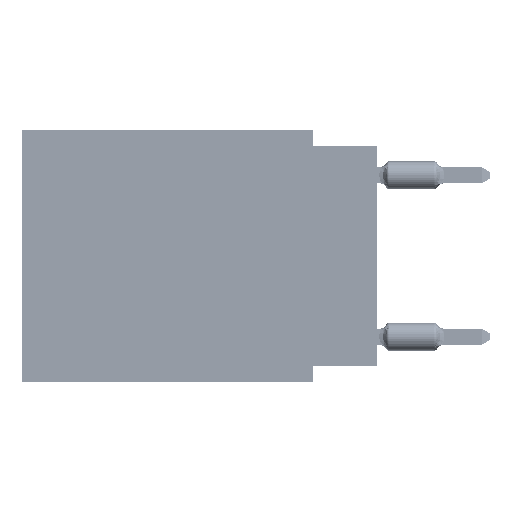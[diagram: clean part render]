
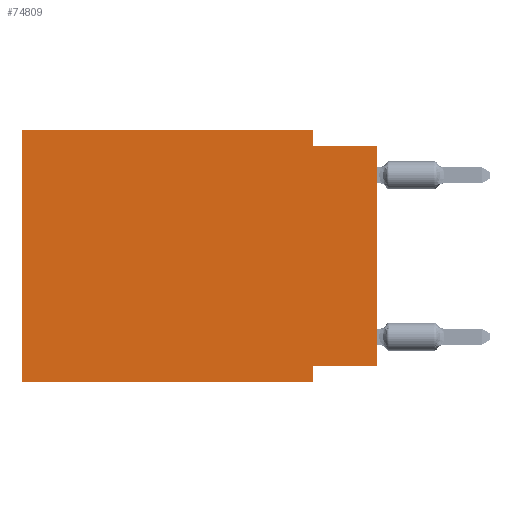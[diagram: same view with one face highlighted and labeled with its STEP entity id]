
A CAD part, left-side view. The second image highlights one B-rep face of the part: STEP entity #74809.
In plain terms, the highlighted planar face has unit normal (-1, 0, 0).
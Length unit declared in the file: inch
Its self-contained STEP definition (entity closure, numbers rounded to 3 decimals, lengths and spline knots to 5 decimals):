
#407 = CARTESIAN_POINT ( 'NONE',  ( 0., 0.1, -0.025 ) ) ;
#1064 = DIRECTION ( 'NONE',  ( 0., -1., 0. ) ) ;
#2382 = LINE ( 'NONE', #27603, #84519 ) ;
#2396 = FACE_OUTER_BOUND ( 'NONE', #12729, .T. ) ;
#2528 = CARTESIAN_POINT ( 'NONE',  ( 0., 0.1, -0.365 ) ) ;
#4672 = VECTOR ( 'NONE', #81144, 39.37008 ) ;
#7283 = CARTESIAN_POINT ( 'NONE',  ( 0., 0.55, -0.39 ) ) ;
#10676 = LINE ( 'NONE', #62419, #72088 ) ;
#12478 = DIRECTION ( 'NONE',  ( 0., -1., 0. ) ) ;
#12547 = VECTOR ( 'NONE', #30053, 39.37008 ) ;
#12703 = CARTESIAN_POINT ( 'NONE',  ( 0., 0.55, 0. ) ) ;
#12729 = EDGE_LOOP ( 'NONE', ( #14983, #24178, #57333, #37853, #65260, #55262, #60399, #20203 ) ) ;
#14983 = ORIENTED_EDGE ( 'NONE', *, *, #69082, .T. ) ;
#19561 = VERTEX_POINT ( 'NONE', #55172 ) ;
#20203 = ORIENTED_EDGE ( 'NONE', *, *, #21071, .F. ) ;
#20659 = PLANE ( 'NONE',  #43314 ) ;
#21071 = EDGE_CURVE ( 'NONE', #53853, #50099, #47751, .T. ) ;
#23182 = VERTEX_POINT ( 'NONE', #60669 ) ;
#24178 = ORIENTED_EDGE ( 'NONE', *, *, #59962, .F. ) ;
#25456 = VERTEX_POINT ( 'NONE', #407 ) ;
#27009 = CARTESIAN_POINT ( 'NONE',  ( 0., 0., -0.365 ) ) ;
#27603 = CARTESIAN_POINT ( 'NONE',  ( 0., 0., 0. ) ) ;
#28454 = EDGE_CURVE ( 'NONE', #53299, #55441, #10676, .T. ) ;
#28886 = DIRECTION ( 'NONE',  ( 1., 0., 0. ) ) ;
#29980 = EDGE_CURVE ( 'NONE', #55441, #23182, #59302, .T. ) ;
#30053 = DIRECTION ( 'NONE',  ( 0., 0., -1. ) ) ;
#30653 = VECTOR ( 'NONE', #1064, 39.37008 ) ;
#30919 = CARTESIAN_POINT ( 'NONE',  ( 0., 0.1, 0. ) ) ;
#37853 = ORIENTED_EDGE ( 'NONE', *, *, #29980, .F. ) ;
#38728 = LINE ( 'NONE', #85182, #50226 ) ;
#43126 = LINE ( 'NONE', #30919, #12547 ) ;
#43314 = AXIS2_PLACEMENT_3D ( 'NONE', #81021, #28886, #81879 ) ;
#43472 = VECTOR ( 'NONE', #12478, 39.37008 ) ;
#47751 = LINE ( 'NONE', #53809, #4672 ) ;
#50099 = VERTEX_POINT ( 'NONE', #2528 ) ;
#50226 = VECTOR ( 'NONE', #53479, 39.37008 ) ;
#53299 = VERTEX_POINT ( 'NONE', #69831 ) ;
#53479 = DIRECTION ( 'NONE',  ( 0., 0., -1. ) ) ;
#53782 = DIRECTION ( 'NONE',  ( 0., -1., 0. ) ) ;
#53809 = CARTESIAN_POINT ( 'NONE',  ( 0., 0., -0.365 ) ) ;
#53853 = VERTEX_POINT ( 'NONE', #27009 ) ;
#54065 = CARTESIAN_POINT ( 'NONE',  ( 0., 0.55, 0. ) ) ;
#55172 = CARTESIAN_POINT ( 'NONE',  ( 0., 0.1, -0.39 ) ) ;
#55262 = ORIENTED_EDGE ( 'NONE', *, *, #78152, .T. ) ;
#55441 = VERTEX_POINT ( 'NONE', #12703 ) ;
#56549 = EDGE_CURVE ( 'NONE', #50099, #19561, #38728, .T. ) ;
#57166 = DIRECTION ( 'NONE',  ( 0., 0., 1. ) ) ;
#57333 = ORIENTED_EDGE ( 'NONE', *, *, #70785, .F. ) ;
#59302 = LINE ( 'NONE', #54065, #30653 ) ;
#59962 = EDGE_CURVE ( 'NONE', #25456, #78010, #84998, .T. ) ;
#60399 = ORIENTED_EDGE ( 'NONE', *, *, #56549, .F. ) ;
#60669 = CARTESIAN_POINT ( 'NONE',  ( 0., 0.1, 0. ) ) ;
#62419 = CARTESIAN_POINT ( 'NONE',  ( 0., 0.55, 0. ) ) ;
#64570 = VECTOR ( 'NONE', #53782, 39.37008 ) ;
#65260 = ORIENTED_EDGE ( 'NONE', *, *, #28454, .F. ) ;
#65468 = CARTESIAN_POINT ( 'NONE',  ( 0., 0., -0.025 ) ) ;
#69082 = EDGE_CURVE ( 'NONE', #53853, #78010, #2382, .T. ) ;
#69831 = CARTESIAN_POINT ( 'NONE',  ( 0., 0.55, -0.39 ) ) ;
#70785 = EDGE_CURVE ( 'NONE', #23182, #25456, #43126, .T. ) ;
#72088 = VECTOR ( 'NONE', #57166, 39.37008 ) ;
#73336 = LINE ( 'NONE', #7283, #64570 ) ;
#74809 = ADVANCED_FACE ( 'NONE', ( #2396 ), #20659, .F. ) ;
#76089 = CARTESIAN_POINT ( 'NONE',  ( 0., 0., -0.025 ) ) ;
#78010 = VERTEX_POINT ( 'NONE', #76089 ) ;
#78152 = EDGE_CURVE ( 'NONE', #53299, #19561, #73336, .T. ) ;
#81021 = CARTESIAN_POINT ( 'NONE',  ( 0., 0.55, 0. ) ) ;
#81144 = DIRECTION ( 'NONE',  ( 0., 1., 0. ) ) ;
#81864 = DIRECTION ( 'NONE',  ( 0., 0., 1. ) ) ;
#81879 = DIRECTION ( 'NONE',  ( 0., 0., -1. ) ) ;
#84519 = VECTOR ( 'NONE', #81864, 39.37008 ) ;
#84998 = LINE ( 'NONE', #65468, #43472 ) ;
#85182 = CARTESIAN_POINT ( 'NONE',  ( 0., 0.1, -0.39 ) ) ;
